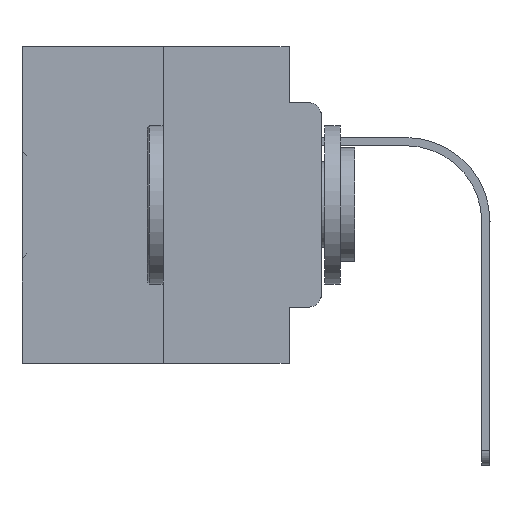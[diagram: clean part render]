
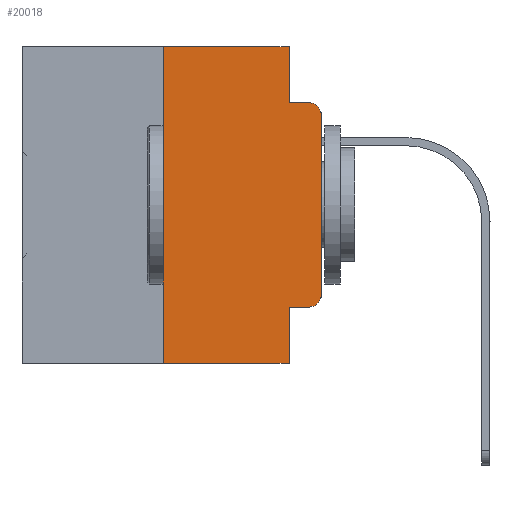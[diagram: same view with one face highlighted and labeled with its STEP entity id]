
A CAD part, left-side view. The second image highlights one B-rep face of the part: STEP entity #20018.
In plain terms, the highlighted planar face has unit normal (-1, 0, 0).
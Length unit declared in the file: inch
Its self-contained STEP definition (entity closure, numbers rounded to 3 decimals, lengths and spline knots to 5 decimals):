
#1072 = DIRECTION ( 'NONE',  ( 0., 0., 1. ) ) ;
#1618 = CARTESIAN_POINT ( 'NONE',  ( 0., 0.051, -0.5 ) ) ;
#2121 = CARTESIAN_POINT ( 'NONE',  ( 0., 0., -0.3915 ) ) ;
#2614 = CARTESIAN_POINT ( 'NONE',  ( 0., 0.051, 0. ) ) ;
#2785 = EDGE_CURVE ( 'NONE', #16456, #10902, #31561, .T. ) ;
#2940 = DIRECTION ( 'NONE',  ( 0., -1., 0. ) ) ;
#3442 = VECTOR ( 'NONE', #15452, 39.37008 ) ;
#3988 = DIRECTION ( 'NONE',  ( -1., 0., 0. ) ) ;
#4159 = CIRCLE ( 'NONE', #16295, 0.02 ) ;
#5358 = EDGE_CURVE ( 'NONE', #12855, #22312, #22704, .T. ) ;
#5491 = CARTESIAN_POINT ( 'NONE',  ( 0., 0.051, 0. ) ) ;
#5495 = EDGE_CURVE ( 'NONE', #22312, #32334, #5696, .T. ) ;
#5696 = LINE ( 'NONE', #18323, #3442 ) ;
#5878 = CARTESIAN_POINT ( 'NONE',  ( 0., 0.051, -0.4115 ) ) ;
#6090 = CARTESIAN_POINT ( 'NONE',  ( 0., 0.051, -0.0885 ) ) ;
#6443 = ORIENTED_EDGE ( 'NONE', *, *, #34027, .T. ) ;
#8015 = ORIENTED_EDGE ( 'NONE', *, *, #27585, .T. ) ;
#8050 = EDGE_CURVE ( 'NONE', #16456, #29609, #29623, .T. ) ;
#8091 = DIRECTION ( 'NONE',  ( 0., 0., -1. ) ) ;
#8183 = DIRECTION ( 'NONE',  ( -1., 0., 0. ) ) ;
#8594 = EDGE_LOOP ( 'NONE', ( #13947, #19520, #31760, #21545, #26719, #20485, #6443, #13003, #24169, #8015 ) ) ;
#9352 = CARTESIAN_POINT ( 'NONE',  ( 0., 0., -0.1085 ) ) ;
#9907 = CARTESIAN_POINT ( 'NONE',  ( 0., 0.051, -0.0885 ) ) ;
#10582 = VECTOR ( 'NONE', #28233, 39.37008 ) ;
#10902 = VERTEX_POINT ( 'NONE', #1618 ) ;
#11508 = VERTEX_POINT ( 'NONE', #16018 ) ;
#11598 = AXIS2_PLACEMENT_3D ( 'NONE', #19894, #3988, #30478 ) ;
#12457 = EDGE_CURVE ( 'NONE', #19293, #18540, #27743, .T. ) ;
#12553 = VERTEX_POINT ( 'NONE', #6090 ) ;
#12674 = VECTOR ( 'NONE', #8091, 39.37008 ) ;
#12855 = VERTEX_POINT ( 'NONE', #32399 ) ;
#13003 = ORIENTED_EDGE ( 'NONE', *, *, #2785, .F. ) ;
#13834 = AXIS2_PLACEMENT_3D ( 'NONE', #14676, #22340, #28189 ) ;
#13843 = EDGE_CURVE ( 'NONE', #18540, #11508, #22120, .T. ) ;
#13947 = ORIENTED_EDGE ( 'NONE', *, *, #12457, .T. ) ;
#14023 = VECTOR ( 'NONE', #28636, 39.37008 ) ;
#14067 = CARTESIAN_POINT ( 'NONE',  ( 0., 0.02, -0.4115 ) ) ;
#14676 = CARTESIAN_POINT ( 'NONE',  ( 0., 0.473, 0. ) ) ;
#15429 = VECTOR ( 'NONE', #33482, 39.37008 ) ;
#15452 = DIRECTION ( 'NONE',  ( 0., -1., 0. ) ) ;
#16018 = CARTESIAN_POINT ( 'NONE',  ( 0., 0.02, -0.0885 ) ) ;
#16295 = AXIS2_PLACEMENT_3D ( 'NONE', #31937, #8183, #18056 ) ;
#16318 = DIRECTION ( 'NONE',  ( 0., 0., -1. ) ) ;
#16456 = VERTEX_POINT ( 'NONE', #21104 ) ;
#17638 = CARTESIAN_POINT ( 'NONE',  ( 0., 0.25, 0. ) ) ;
#17814 = VECTOR ( 'NONE', #16318, 39.37008 ) ;
#17865 = EDGE_CURVE ( 'NONE', #32334, #12553, #29524, .T. ) ;
#18056 = DIRECTION ( 'NONE',  ( 0., 0., -1. ) ) ;
#18323 = CARTESIAN_POINT ( 'NONE',  ( 0., 0.473, 0. ) ) ;
#18540 = VERTEX_POINT ( 'NONE', #9352 ) ;
#19293 = VERTEX_POINT ( 'NONE', #2121 ) ;
#19520 = ORIENTED_EDGE ( 'NONE', *, *, #13843, .T. ) ;
#19894 = CARTESIAN_POINT ( 'NONE',  ( 0., 0.02, -0.1085 ) ) ;
#20018 = ADVANCED_FACE ( 'NONE', ( #30964 ), #33427, .F. ) ;
#20485 = ORIENTED_EDGE ( 'NONE', *, *, #5358, .F. ) ;
#21104 = CARTESIAN_POINT ( 'NONE',  ( 0., 0.051, -0.4115 ) ) ;
#21545 = ORIENTED_EDGE ( 'NONE', *, *, #17865, .F. ) ;
#22120 = CIRCLE ( 'NONE', #11598, 0.02 ) ;
#22312 = VERTEX_POINT ( 'NONE', #24410 ) ;
#22340 = DIRECTION ( 'NONE',  ( 1., 0., 0. ) ) ;
#22704 = LINE ( 'NONE', #17638, #10582 ) ;
#23402 = LINE ( 'NONE', #30858, #15429 ) ;
#23430 = EDGE_CURVE ( 'NONE', #12553, #11508, #25513, .T. ) ;
#24169 = ORIENTED_EDGE ( 'NONE', *, *, #8050, .T. ) ;
#24410 = CARTESIAN_POINT ( 'NONE',  ( 0., 0.25, 0. ) ) ;
#24651 = CARTESIAN_POINT ( 'NONE',  ( 0., 0., 0. ) ) ;
#24690 = VECTOR ( 'NONE', #1072, 39.37008 ) ;
#25513 = LINE ( 'NONE', #9907, #14023 ) ;
#25606 = VECTOR ( 'NONE', #2940, 39.37008 ) ;
#26719 = ORIENTED_EDGE ( 'NONE', *, *, #5495, .F. ) ;
#27086 = CARTESIAN_POINT ( 'NONE',  ( 0., 0.051, 0. ) ) ;
#27585 = EDGE_CURVE ( 'NONE', #29609, #19293, #4159, .T. ) ;
#27743 = LINE ( 'NONE', #24651, #24690 ) ;
#28189 = DIRECTION ( 'NONE',  ( 0., 0., -1. ) ) ;
#28233 = DIRECTION ( 'NONE',  ( 0., 0., 1. ) ) ;
#28636 = DIRECTION ( 'NONE',  ( 0., -1., 0. ) ) ;
#29524 = LINE ( 'NONE', #27086, #17814 ) ;
#29609 = VERTEX_POINT ( 'NONE', #14067 ) ;
#29623 = LINE ( 'NONE', #5878, #25606 ) ;
#30478 = DIRECTION ( 'NONE',  ( 0., 0., -1. ) ) ;
#30858 = CARTESIAN_POINT ( 'NONE',  ( 0., 0.473, -0.5 ) ) ;
#30964 = FACE_OUTER_BOUND ( 'NONE', #8594, .T. ) ;
#31561 = LINE ( 'NONE', #5491, #12674 ) ;
#31760 = ORIENTED_EDGE ( 'NONE', *, *, #23430, .F. ) ;
#31937 = CARTESIAN_POINT ( 'NONE',  ( 0., 0.02, -0.3915 ) ) ;
#32334 = VERTEX_POINT ( 'NONE', #2614 ) ;
#32399 = CARTESIAN_POINT ( 'NONE',  ( 0., 0.25, -0.5 ) ) ;
#33427 = PLANE ( 'NONE',  #13834 ) ;
#33482 = DIRECTION ( 'NONE',  ( 0., -1., 0. ) ) ;
#34027 = EDGE_CURVE ( 'NONE', #12855, #10902, #23402, .T. ) ;
